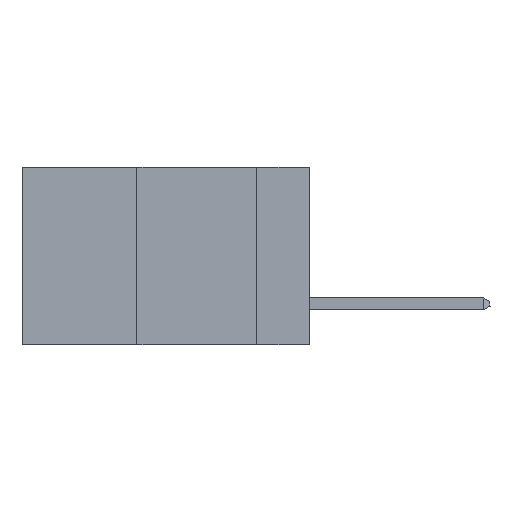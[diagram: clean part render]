
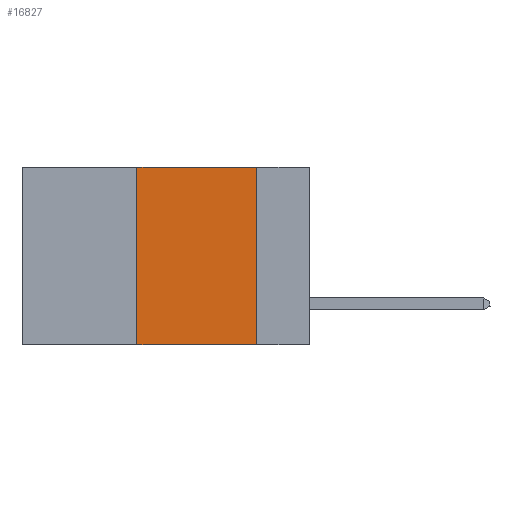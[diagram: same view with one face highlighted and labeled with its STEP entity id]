
A CAD part, left-side view. The second image highlights one B-rep face of the part: STEP entity #16827.
In plain terms, the highlighted planar face has unit normal (-1, 0, 0).
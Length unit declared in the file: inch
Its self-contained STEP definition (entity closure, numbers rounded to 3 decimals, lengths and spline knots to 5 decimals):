
#157 = EDGE_CURVE ( 'NONE', #6588, #14653, #15907, .T. ) ;
#548 = VECTOR ( 'NONE', #21232, 39.37008 ) ;
#880 = ORIENTED_EDGE ( 'NONE', *, *, #942, .F. ) ;
#899 = CARTESIAN_POINT ( 'NONE',  ( 0., 0.6, -0.37 ) ) ;
#942 = EDGE_CURVE ( 'NONE', #16424, #14653, #17097, .T. ) ;
#1568 = LINE ( 'NONE', #22777, #12860 ) ;
#2256 = ORIENTED_EDGE ( 'NONE', *, *, #11399, .F. ) ;
#3078 = EDGE_LOOP ( 'NONE', ( #880, #22095, #2256, #12494 ) ) ;
#3434 = VERTEX_POINT ( 'NONE', #18053 ) ;
#6588 = VERTEX_POINT ( 'NONE', #6615 ) ;
#6615 = CARTESIAN_POINT ( 'NONE',  ( 0., 0.36, -0.37 ) ) ;
#7560 = VECTOR ( 'NONE', #22930, 39.37008 ) ;
#8756 = FACE_OUTER_BOUND ( 'NONE', #3078, .T. ) ;
#9082 = EDGE_CURVE ( 'NONE', #3434, #16424, #14650, .T. ) ;
#10841 = CARTESIAN_POINT ( 'NONE',  ( 0., 0.11, 0. ) ) ;
#10946 = DIRECTION ( 'NONE',  ( 0., 0., -1. ) ) ;
#11399 = EDGE_CURVE ( 'NONE', #6588, #3434, #1568, .T. ) ;
#12494 = ORIENTED_EDGE ( 'NONE', *, *, #157, .T. ) ;
#12860 = VECTOR ( 'NONE', #26646, 39.37008 ) ;
#14502 = CARTESIAN_POINT ( 'NONE',  ( 0., 0.6, 0. ) ) ;
#14650 = LINE ( 'NONE', #14502, #7560 ) ;
#14653 = VERTEX_POINT ( 'NONE', #24797 ) ;
#15082 = CARTESIAN_POINT ( 'NONE',  ( 0., 0.6, 0. ) ) ;
#15356 = PLANE ( 'NONE',  #22702 ) ;
#15907 = LINE ( 'NONE', #899, #20748 ) ;
#16424 = VERTEX_POINT ( 'NONE', #10841 ) ;
#16827 = ADVANCED_FACE ( 'NONE', ( #8756 ), #15356, .F. ) ;
#17097 = LINE ( 'NONE', #27153, #548 ) ;
#18053 = CARTESIAN_POINT ( 'NONE',  ( 0., 0.36, 0. ) ) ;
#20748 = VECTOR ( 'NONE', #21709, 39.37008 ) ;
#21232 = DIRECTION ( 'NONE',  ( 0., 0., -1. ) ) ;
#21709 = DIRECTION ( 'NONE',  ( 0., -1., 0. ) ) ;
#22095 = ORIENTED_EDGE ( 'NONE', *, *, #9082, .F. ) ;
#22702 = AXIS2_PLACEMENT_3D ( 'NONE', #15082, #23500, #10946 ) ;
#22777 = CARTESIAN_POINT ( 'NONE',  ( 0., 0.36, 0. ) ) ;
#22930 = DIRECTION ( 'NONE',  ( 0., -1., 0. ) ) ;
#23500 = DIRECTION ( 'NONE',  ( 1., 0., 0. ) ) ;
#24797 = CARTESIAN_POINT ( 'NONE',  ( 0., 0.11, -0.37 ) ) ;
#26646 = DIRECTION ( 'NONE',  ( 0., 0., 1. ) ) ;
#27153 = CARTESIAN_POINT ( 'NONE',  ( 0., 0.11, 0. ) ) ;
